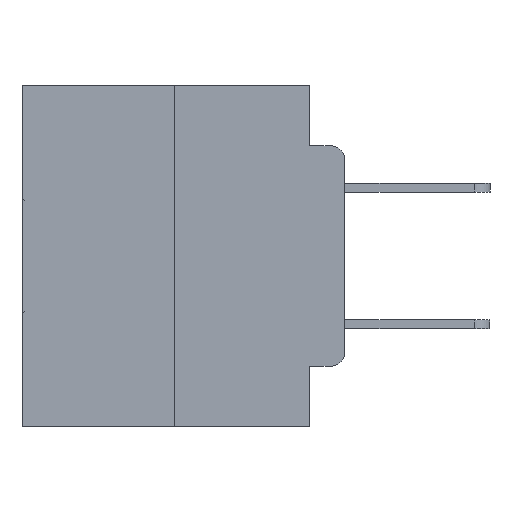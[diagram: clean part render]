
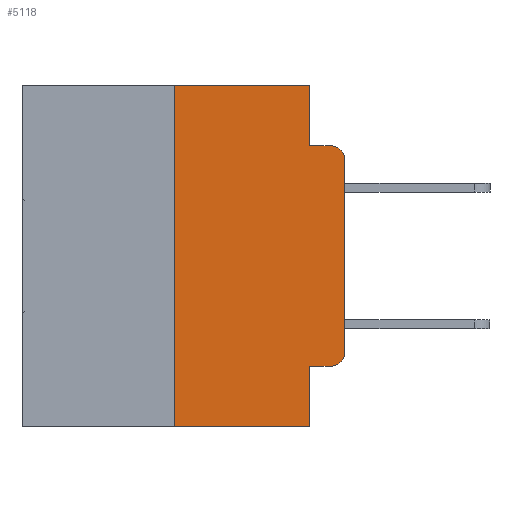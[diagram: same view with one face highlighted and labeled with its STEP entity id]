
A CAD part, left-side view. The second image highlights one B-rep face of the part: STEP entity #5118.
In plain terms, the highlighted planar face has unit normal (-1, 0, 0).
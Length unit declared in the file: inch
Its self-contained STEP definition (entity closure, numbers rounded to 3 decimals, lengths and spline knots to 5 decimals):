
#459 = VERTEX_POINT ( 'NONE', #13169 ) ;
#699 = CARTESIAN_POINT ( 'NONE',  ( 0., 0.051, 0. ) ) ;
#846 = EDGE_CURVE ( 'NONE', #19818, #20814, #1108, .T. ) ;
#976 = ORIENTED_EDGE ( 'NONE', *, *, #29368, .T. ) ;
#1108 = LINE ( 'NONE', #22755, #19027 ) ;
#1642 = AXIS2_PLACEMENT_3D ( 'NONE', #5424, #21631, #7780 ) ;
#3183 = VECTOR ( 'NONE', #10604, 39.37008 ) ;
#3597 = FACE_OUTER_BOUND ( 'NONE', #24791, .T. ) ;
#3646 = CARTESIAN_POINT ( 'NONE',  ( 0., 0.473, 0. ) ) ;
#3690 = CIRCLE ( 'NONE', #17230, 0.02 ) ;
#4898 = CARTESIAN_POINT ( 'NONE',  ( 0., 0.25, -0.5 ) ) ;
#5118 = ADVANCED_FACE ( 'NONE', ( #3597 ), #7078, .F. ) ;
#5424 = CARTESIAN_POINT ( 'NONE',  ( 0., 0.02, -0.1085 ) ) ;
#5716 = CARTESIAN_POINT ( 'NONE',  ( 0., 0.051, -0.5 ) ) ;
#5982 = DIRECTION ( 'NONE',  ( 1., 0., 0. ) ) ;
#6176 = ORIENTED_EDGE ( 'NONE', *, *, #10943, .T. ) ;
#6638 = LINE ( 'NONE', #14799, #24377 ) ;
#6654 = DIRECTION ( 'NONE',  ( 0., 0., 1. ) ) ;
#6687 = DIRECTION ( 'NONE',  ( -1., 0., 0. ) ) ;
#7078 = PLANE ( 'NONE',  #28994 ) ;
#7780 = DIRECTION ( 'NONE',  ( 0., 0., -1. ) ) ;
#8975 = DIRECTION ( 'NONE',  ( 0., -1., 0. ) ) ;
#9443 = LINE ( 'NONE', #10407, #3183 ) ;
#10225 = DIRECTION ( 'NONE',  ( 0., 0., 1. ) ) ;
#10407 = CARTESIAN_POINT ( 'NONE',  ( 0., 0.051, -0.0885 ) ) ;
#10604 = DIRECTION ( 'NONE',  ( 0., -1., 0. ) ) ;
#10737 = VECTOR ( 'NONE', #22231, 39.37008 ) ;
#10943 = EDGE_CURVE ( 'NONE', #25807, #14144, #3690, .T. ) ;
#11852 = VERTEX_POINT ( 'NONE', #17245 ) ;
#12024 = ORIENTED_EDGE ( 'NONE', *, *, #18212, .F. ) ;
#12137 = VECTOR ( 'NONE', #17089, 39.37008 ) ;
#12584 = CARTESIAN_POINT ( 'NONE',  ( 0., 0., 0. ) ) ;
#12928 = LINE ( 'NONE', #3646, #10737 ) ;
#13169 = CARTESIAN_POINT ( 'NONE',  ( 0., 0.051, -0.0885 ) ) ;
#13444 = CARTESIAN_POINT ( 'NONE',  ( 0., 0.051, -0.4115 ) ) ;
#13666 = CARTESIAN_POINT ( 'NONE',  ( 0., 0.473, 0. ) ) ;
#14144 = VERTEX_POINT ( 'NONE', #14513 ) ;
#14240 = ORIENTED_EDGE ( 'NONE', *, *, #29383, .F. ) ;
#14513 = CARTESIAN_POINT ( 'NONE',  ( 0., 0., -0.3915 ) ) ;
#14799 = CARTESIAN_POINT ( 'NONE',  ( 0., 0.473, -0.5 ) ) ;
#15201 = CARTESIAN_POINT ( 'NONE',  ( 0., 0.051, 0. ) ) ;
#15331 = ORIENTED_EDGE ( 'NONE', *, *, #26599, .T. ) ;
#15402 = VERTEX_POINT ( 'NONE', #5716 ) ;
#15626 = EDGE_CURVE ( 'NONE', #25043, #25807, #26349, .T. ) ;
#15846 = CARTESIAN_POINT ( 'NONE',  ( 0., 0.051, 0. ) ) ;
#17089 = DIRECTION ( 'NONE',  ( 0., 0., -1. ) ) ;
#17230 = AXIS2_PLACEMENT_3D ( 'NONE', #20598, #6687, #22879 ) ;
#17245 = CARTESIAN_POINT ( 'NONE',  ( 0., 0., -0.1085 ) ) ;
#18199 = ORIENTED_EDGE ( 'NONE', *, *, #846, .F. ) ;
#18212 = EDGE_CURVE ( 'NONE', #20814, #29483, #12928, .T. ) ;
#18232 = CARTESIAN_POINT ( 'NONE',  ( 0., 0.02, -0.4115 ) ) ;
#18233 = CARTESIAN_POINT ( 'NONE',  ( 0., 0.051, -0.4115 ) ) ;
#18256 = LINE ( 'NONE', #12584, #29659 ) ;
#18972 = CARTESIAN_POINT ( 'NONE',  ( 0., 0.02, -0.0885 ) ) ;
#19010 = LINE ( 'NONE', #699, #12137 ) ;
#19027 = VECTOR ( 'NONE', #6654, 39.37008 ) ;
#19818 = VERTEX_POINT ( 'NONE', #4898 ) ;
#20298 = VECTOR ( 'NONE', #8975, 39.37008 ) ;
#20598 = CARTESIAN_POINT ( 'NONE',  ( 0., 0.02, -0.3915 ) ) ;
#20814 = VERTEX_POINT ( 'NONE', #26288 ) ;
#21358 = EDGE_CURVE ( 'NONE', #11852, #29932, #29942, .T. ) ;
#21631 = DIRECTION ( 'NONE',  ( -1., 0., 0. ) ) ;
#22231 = DIRECTION ( 'NONE',  ( 0., -1., 0. ) ) ;
#22755 = CARTESIAN_POINT ( 'NONE',  ( 0., 0.25, 0. ) ) ;
#22829 = ORIENTED_EDGE ( 'NONE', *, *, #27317, .F. ) ;
#22879 = DIRECTION ( 'NONE',  ( 0., 0., -1. ) ) ;
#23184 = ORIENTED_EDGE ( 'NONE', *, *, #15626, .T. ) ;
#24377 = VECTOR ( 'NONE', #28474, 39.37008 ) ;
#24707 = LINE ( 'NONE', #15846, #30010 ) ;
#24791 = EDGE_LOOP ( 'NONE', ( #15331, #27474, #22829, #29598, #12024, #18199, #976, #14240, #23184, #6176 ) ) ;
#25043 = VERTEX_POINT ( 'NONE', #13444 ) ;
#25764 = EDGE_CURVE ( 'NONE', #29483, #459, #24707, .T. ) ;
#25807 = VERTEX_POINT ( 'NONE', #18232 ) ;
#26288 = CARTESIAN_POINT ( 'NONE',  ( 0., 0.25, 0. ) ) ;
#26349 = LINE ( 'NONE', #18233, #20298 ) ;
#26599 = EDGE_CURVE ( 'NONE', #14144, #11852, #18256, .T. ) ;
#27317 = EDGE_CURVE ( 'NONE', #459, #29932, #9443, .T. ) ;
#27474 = ORIENTED_EDGE ( 'NONE', *, *, #21358, .T. ) ;
#28331 = DIRECTION ( 'NONE',  ( 0., 0., -1. ) ) ;
#28474 = DIRECTION ( 'NONE',  ( 0., -1., 0. ) ) ;
#28994 = AXIS2_PLACEMENT_3D ( 'NONE', #13666, #5982, #28331 ) ;
#29368 = EDGE_CURVE ( 'NONE', #19818, #15402, #6638, .T. ) ;
#29383 = EDGE_CURVE ( 'NONE', #25043, #15402, #19010, .T. ) ;
#29483 = VERTEX_POINT ( 'NONE', #15201 ) ;
#29491 = DIRECTION ( 'NONE',  ( 0., 0., -1. ) ) ;
#29598 = ORIENTED_EDGE ( 'NONE', *, *, #25764, .F. ) ;
#29659 = VECTOR ( 'NONE', #10225, 39.37008 ) ;
#29932 = VERTEX_POINT ( 'NONE', #18972 ) ;
#29942 = CIRCLE ( 'NONE', #1642, 0.02 ) ;
#30010 = VECTOR ( 'NONE', #29491, 39.37008 ) ;
